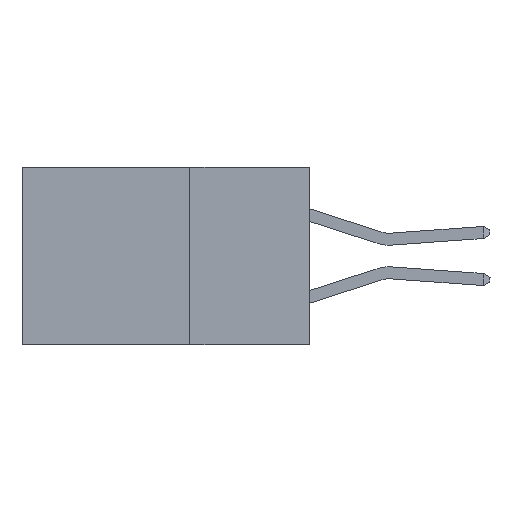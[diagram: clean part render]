
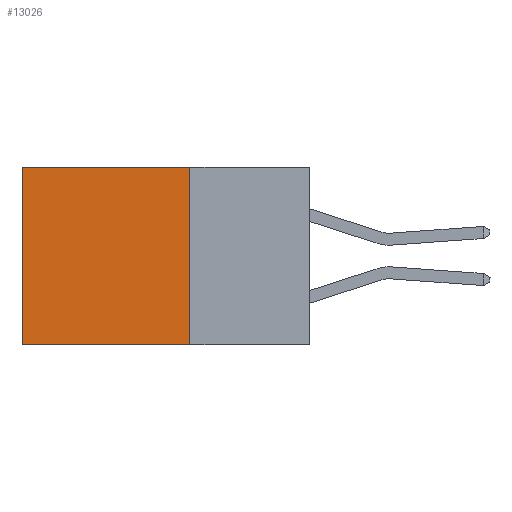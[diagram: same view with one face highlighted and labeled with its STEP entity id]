
A CAD part, left-side view. The second image highlights one B-rep face of the part: STEP entity #13026.
In plain terms, the highlighted planar face has unit normal (-1, 0, 0).
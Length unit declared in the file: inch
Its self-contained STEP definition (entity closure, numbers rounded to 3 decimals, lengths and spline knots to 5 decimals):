
#182 = DIRECTION ( 'NONE',  ( 0., 0., -1. ) ) ;
#987 = VERTEX_POINT ( 'NONE', #16284 ) ;
#1052 = LINE ( 'NONE', #23301, #25762 ) ;
#1098 = DIRECTION ( 'NONE',  ( 0., 0., -1. ) ) ;
#1183 = LINE ( 'NONE', #13642, #23636 ) ;
#1328 = FACE_OUTER_BOUND ( 'NONE', #10256, .T. ) ;
#2124 = DIRECTION ( 'NONE',  ( 1., 0., 0. ) ) ;
#3771 = CARTESIAN_POINT ( 'NONE',  ( 0.298, 0.25, 0. ) ) ;
#4166 = DIRECTION ( 'NONE',  ( 0., 0., -1. ) ) ;
#5327 = ORIENTED_EDGE ( 'NONE', *, *, #16465, .T. ) ;
#6141 = CARTESIAN_POINT ( 'NONE',  ( 0.298, 0.25, 0. ) ) ;
#6445 = PLANE ( 'NONE',  #15776 ) ;
#6598 = CARTESIAN_POINT ( 'NONE',  ( 0.298, 0.6, 0. ) ) ;
#8138 = ORIENTED_EDGE ( 'NONE', *, *, #24770, .T. ) ;
#9071 = ORIENTED_EDGE ( 'NONE', *, *, #15626, .F. ) ;
#9138 = ORIENTED_EDGE ( 'NONE', *, *, #23669, .F. ) ;
#10256 = EDGE_LOOP ( 'NONE', ( #5327, #9071, #9138, #8138 ) ) ;
#10281 = VERTEX_POINT ( 'NONE', #3771 ) ;
#11817 = VERTEX_POINT ( 'NONE', #12473 ) ;
#12473 = CARTESIAN_POINT ( 'NONE',  ( 0.298, 0.25, -0.37 ) ) ;
#12913 = LINE ( 'NONE', #6141, #14809 ) ;
#13026 = ADVANCED_FACE ( 'NONE', ( #1328 ), #6445, .F. ) ;
#13642 = CARTESIAN_POINT ( 'NONE',  ( 0.298, 0.25, -0.37 ) ) ;
#14809 = VECTOR ( 'NONE', #16407, 39.37008 ) ;
#15626 = EDGE_CURVE ( 'NONE', #11817, #987, #1183, .T. ) ;
#15776 = AXIS2_PLACEMENT_3D ( 'NONE', #24345, #2124, #4166 ) ;
#16230 = CARTESIAN_POINT ( 'NONE',  ( 0.298, 0.25, 0. ) ) ;
#16284 = CARTESIAN_POINT ( 'NONE',  ( 0.298, 0.6, -0.37 ) ) ;
#16407 = DIRECTION ( 'NONE',  ( 0., 1., 0. ) ) ;
#16465 = EDGE_CURVE ( 'NONE', #19281, #987, #1052, .T. ) ;
#19281 = VERTEX_POINT ( 'NONE', #6598 ) ;
#20921 = VECTOR ( 'NONE', #182, 39.37008 ) ;
#21543 = DIRECTION ( 'NONE',  ( 0., 1., 0. ) ) ;
#22819 = LINE ( 'NONE', #16230, #20921 ) ;
#23301 = CARTESIAN_POINT ( 'NONE',  ( 0.298, 0.6, 0. ) ) ;
#23636 = VECTOR ( 'NONE', #21543, 39.37008 ) ;
#23669 = EDGE_CURVE ( 'NONE', #10281, #11817, #22819, .T. ) ;
#24345 = CARTESIAN_POINT ( 'NONE',  ( 0.298, 0.25, 0. ) ) ;
#24770 = EDGE_CURVE ( 'NONE', #10281, #19281, #12913, .T. ) ;
#25762 = VECTOR ( 'NONE', #1098, 39.37008 ) ;
